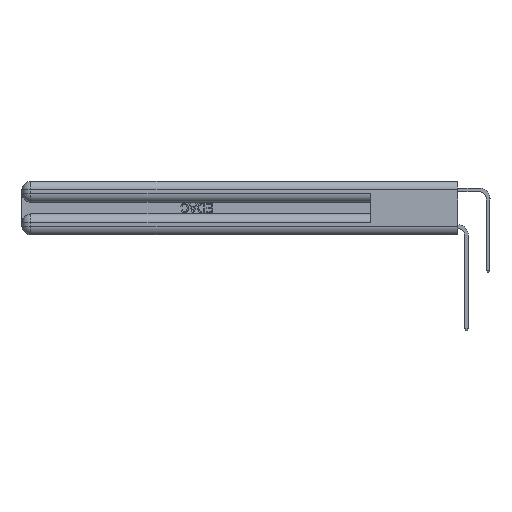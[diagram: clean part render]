
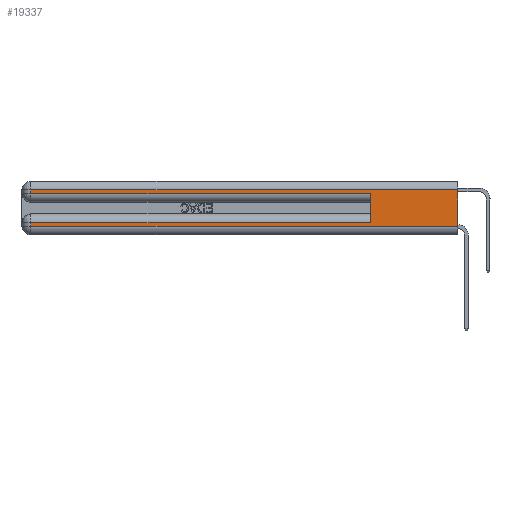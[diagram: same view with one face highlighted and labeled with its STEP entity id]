
A CAD part, left-side view. The second image highlights one B-rep face of the part: STEP entity #19337.
In plain terms, the highlighted planar face has unit normal (-1, 0, 0).
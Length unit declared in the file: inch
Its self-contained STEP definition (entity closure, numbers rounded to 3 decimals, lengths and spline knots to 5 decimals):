
#373 = EDGE_CURVE ( 'NONE', #27075, #23266, #34174, .T. ) ;
#626 = CARTESIAN_POINT ( 'NONE',  ( 0., 2.94, 0.31 ) ) ;
#1192 = VECTOR ( 'NONE', #30104, 39.37008 ) ;
#1384 = FACE_OUTER_BOUND ( 'NONE', #2245, .T. ) ;
#2132 = EDGE_CURVE ( 'NONE', #23266, #18516, #23140, .T. ) ;
#2245 = EDGE_LOOP ( 'NONE', ( #2512, #12659, #33952, #3754, #19775, #3459, #26966, #26952 ) ) ;
#2470 = DIRECTION ( 'NONE',  ( 0., 1., 0. ) ) ;
#2512 = ORIENTED_EDGE ( 'NONE', *, *, #24927, .F. ) ;
#2781 = DIRECTION ( 'NONE',  ( 0., 1., 0. ) ) ;
#3459 = ORIENTED_EDGE ( 'NONE', *, *, #9669, .T. ) ;
#3610 = CARTESIAN_POINT ( 'NONE',  ( 0., 0., 0.31 ) ) ;
#3754 = ORIENTED_EDGE ( 'NONE', *, *, #2132, .T. ) ;
#3943 = CARTESIAN_POINT ( 'NONE',  ( 0., 2.94, 0.37 ) ) ;
#4304 = CARTESIAN_POINT ( 'NONE',  ( 0., 0., 0.37 ) ) ;
#5221 = DIRECTION ( 'NONE',  ( 0., 0., 1. ) ) ;
#6681 = CARTESIAN_POINT ( 'NONE',  ( 0., 0.6, 0.085 ) ) ;
#8001 = VECTOR ( 'NONE', #13472, 39.37008 ) ;
#8332 = CARTESIAN_POINT ( 'NONE',  ( 0., 0., 0.37 ) ) ;
#8365 = VERTEX_POINT ( 'NONE', #24394 ) ;
#9669 = EDGE_CURVE ( 'NONE', #12366, #8365, #32489, .T. ) ;
#12039 = LINE ( 'NONE', #18154, #1192 ) ;
#12366 = VERTEX_POINT ( 'NONE', #6681 ) ;
#12659 = ORIENTED_EDGE ( 'NONE', *, *, #14569, .T. ) ;
#12897 = DIRECTION ( 'NONE',  ( 0., -1., 0. ) ) ;
#13472 = DIRECTION ( 'NONE',  ( 0., 0., -1. ) ) ;
#13506 = VECTOR ( 'NONE', #2470, 39.37008 ) ;
#14339 = CARTESIAN_POINT ( 'NONE',  ( 0., 0., 0.085 ) ) ;
#14416 = DIRECTION ( 'NONE',  ( 0., 0., -1. ) ) ;
#14569 = EDGE_CURVE ( 'NONE', #16325, #27075, #20091, .T. ) ;
#15596 = EDGE_CURVE ( 'NONE', #32872, #31272, #12039, .T. ) ;
#16214 = VECTOR ( 'NONE', #2781, 39.37008 ) ;
#16325 = VERTEX_POINT ( 'NONE', #3610 ) ;
#17232 = CARTESIAN_POINT ( 'NONE',  ( 0., 0.6, 0.145 ) ) ;
#18034 = VECTOR ( 'NONE', #12897, 39.37008 ) ;
#18154 = CARTESIAN_POINT ( 'NONE',  ( 0., 0., 0.06 ) ) ;
#18274 = VECTOR ( 'NONE', #5221, 39.37008 ) ;
#18516 = VERTEX_POINT ( 'NONE', #23725 ) ;
#19337 = ADVANCED_FACE ( 'NONE', ( #1384 ), #29026, .F. ) ;
#19775 = ORIENTED_EDGE ( 'NONE', *, *, #22409, .F. ) ;
#20091 = LINE ( 'NONE', #20184, #13506 ) ;
#20184 = CARTESIAN_POINT ( 'NONE',  ( 0., 0., 0.31 ) ) ;
#20509 = AXIS2_PLACEMENT_3D ( 'NONE', #8332, #26222, #29275 ) ;
#22082 = CARTESIAN_POINT ( 'NONE',  ( 0., 2.94, 0.37 ) ) ;
#22409 = EDGE_CURVE ( 'NONE', #12366, #18516, #26120, .T. ) ;
#23140 = LINE ( 'NONE', #24665, #18034 ) ;
#23195 = EDGE_CURVE ( 'NONE', #8365, #32872, #37726, .T. ) ;
#23266 = VERTEX_POINT ( 'NONE', #25211 ) ;
#23725 = CARTESIAN_POINT ( 'NONE',  ( 0., 0.6, 0.285 ) ) ;
#24394 = CARTESIAN_POINT ( 'NONE',  ( 0., 2.94, 0.085 ) ) ;
#24665 = CARTESIAN_POINT ( 'NONE',  ( 0., 0., 0.285 ) ) ;
#24927 = EDGE_CURVE ( 'NONE', #16325, #31272, #30662, .T. ) ;
#25052 = DIRECTION ( 'NONE',  ( 0., 0., -1. ) ) ;
#25211 = CARTESIAN_POINT ( 'NONE',  ( 0., 2.94, 0.285 ) ) ;
#25792 = VECTOR ( 'NONE', #25052, 39.37008 ) ;
#26120 = LINE ( 'NONE', #17232, #18274 ) ;
#26222 = DIRECTION ( 'NONE',  ( 1., 0., 0. ) ) ;
#26952 = ORIENTED_EDGE ( 'NONE', *, *, #15596, .T. ) ;
#26966 = ORIENTED_EDGE ( 'NONE', *, *, #23195, .T. ) ;
#27075 = VERTEX_POINT ( 'NONE', #626 ) ;
#29026 = PLANE ( 'NONE',  #20509 ) ;
#29275 = DIRECTION ( 'NONE',  ( 0., 0., -1. ) ) ;
#30104 = DIRECTION ( 'NONE',  ( 0., -1., 0. ) ) ;
#30662 = LINE ( 'NONE', #4304, #31567 ) ;
#31272 = VERTEX_POINT ( 'NONE', #35779 ) ;
#31567 = VECTOR ( 'NONE', #14416, 39.37008 ) ;
#32489 = LINE ( 'NONE', #14339, #16214 ) ;
#32872 = VERTEX_POINT ( 'NONE', #37125 ) ;
#33952 = ORIENTED_EDGE ( 'NONE', *, *, #373, .T. ) ;
#34174 = LINE ( 'NONE', #3943, #25792 ) ;
#35779 = CARTESIAN_POINT ( 'NONE',  ( 0., 0., 0.06 ) ) ;
#37125 = CARTESIAN_POINT ( 'NONE',  ( 0., 2.94, 0.06 ) ) ;
#37726 = LINE ( 'NONE', #22082, #8001 ) ;
